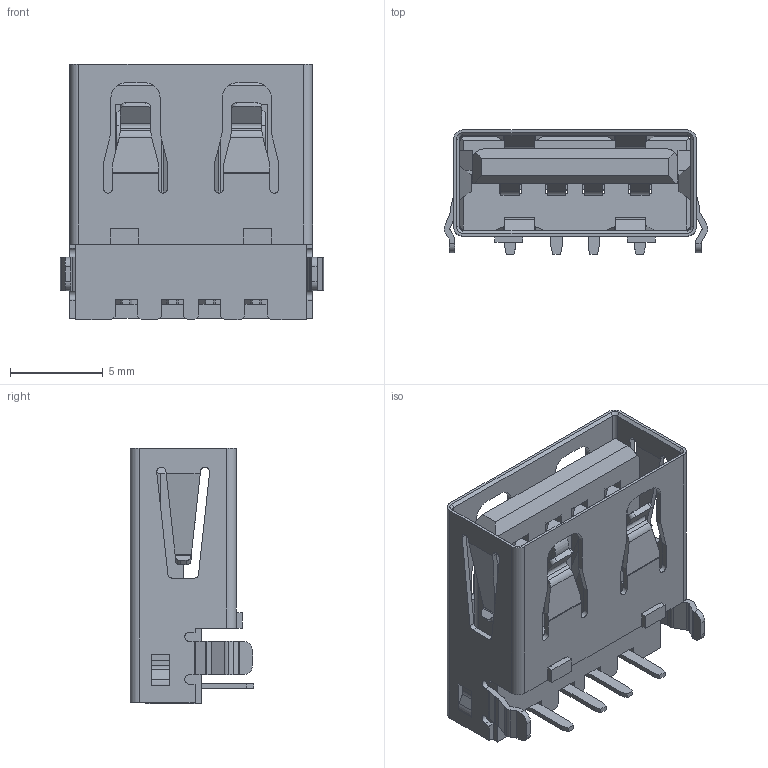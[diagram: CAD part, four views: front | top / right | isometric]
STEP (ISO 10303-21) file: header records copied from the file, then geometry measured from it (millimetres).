
FILE_DESCRIPTION (( 'STEP AP214' ), '1' );
FILE_NAME ('690G104-253-221.STEP', '2021-01-14T12:57:25', ( '' ), ( '' ), 'SwSTEP 2.0', 'SolidWorks 2020', '' );
FILE_SCHEMA (( 'AUTOMOTIVE_DESIGN' ));
Length unit declared in the file: millimetre
Products named in the file (4): Shell 690G104-253-22X; Contact 690G104-253-22X; Insulator 690G104-253-22X_Black; 690G104-253-221
Assembly tree (6 placements, depth 2):
  690G104-253-221
    Insulator 690G104-253-22X_Black
    Contact 690G104-253-22X  x4
    Shell 690G104-253-22X
Bounding box: 14.2 x 6.67 x 13.78 mm (x, y, z)
Volume: 406.6 mm3; surface area: 1711.7 mm2
Topology: 6 solids, 6 shells, 738 faces, 2130 edges, 1395 vertices
Faces by surface type: plane 554, cylinder 164, bspline 16, cone 4
Entity records: 18808 total; most frequent: CARTESIAN_POINT 4043, ORIENTED_EDGE 3198, DIRECTION 2861, EDGE_CURVE 1599, VECTOR 1273, LINE 1273, VERTEX_POINT 1041, AXIS2_PLACEMENT_3D 794
